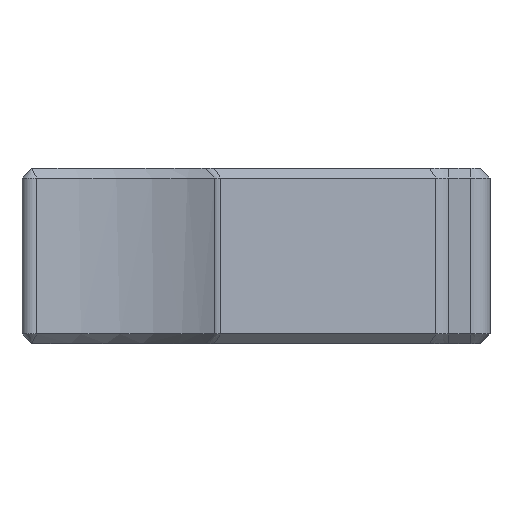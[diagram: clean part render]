
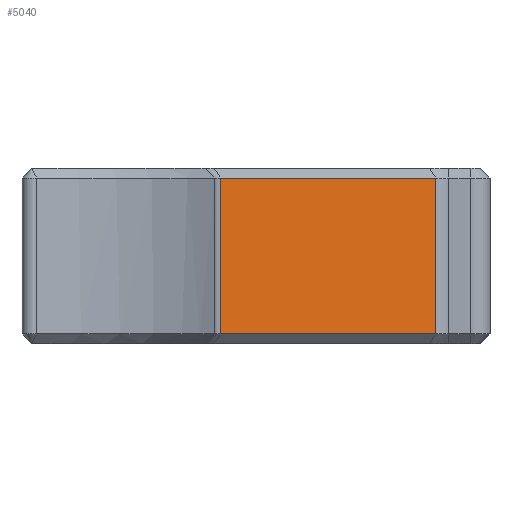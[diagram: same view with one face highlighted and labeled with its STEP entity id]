
A CAD part, front view. The second image highlights one B-rep face of the part: STEP entity #5040.
In plain terms, the highlighted planar face has unit normal (0.658, -0.753, 0).
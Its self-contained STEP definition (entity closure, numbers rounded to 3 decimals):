
#295 = VERTEX_POINT ( 'NONE', #6923 ) ;
#414 = EDGE_CURVE ( 'NONE', #295, #7731, #649, .T. ) ;
#551 = EDGE_LOOP ( 'NONE', ( #2454, #8305, #5130, #1067 ) ) ;
#649 = LINE ( 'NONE', #7793, #1592 ) ;
#946 = DIRECTION ( 'NONE',  ( -0.753, -0.658, 0. ) ) ;
#1033 = EDGE_CURVE ( 'NONE', #1755, #295, #6708, .T. ) ;
#1067 = ORIENTED_EDGE ( 'NONE', *, *, #8392, .T. ) ;
#1592 = VECTOR ( 'NONE', #3863, 1000. ) ;
#1755 = VERTEX_POINT ( 'NONE', #3009 ) ;
#1832 = CARTESIAN_POINT ( 'NONE',  ( 8.379, -9.581, -4. ) ) ;
#2094 = VECTOR ( 'NONE', #2822, 1000. ) ;
#2454 = ORIENTED_EDGE ( 'NONE', *, *, #7934, .T. ) ;
#2777 = DIRECTION ( 'NONE',  ( -0.658, 0.753, 0. ) ) ;
#2822 = DIRECTION ( 'NONE',  ( 0., 0., -1. ) ) ;
#3009 = CARTESIAN_POINT ( 'NONE',  ( 3.688, -13.683, -4. ) ) ;
#3605 = CARTESIAN_POINT ( 'NONE',  ( 3.688, -13.683, 4.5 ) ) ;
#3608 = CARTESIAN_POINT ( 'NONE',  ( 8.379, -9.581, 4.5 ) ) ;
#3863 = DIRECTION ( 'NONE',  ( 0., 0., 1. ) ) ;
#4887 = CARTESIAN_POINT ( 'NONE',  ( 3.688, -13.683, 4. ) ) ;
#5040 = ADVANCED_FACE ( 'NONE', ( #6718 ), #7538, .F. ) ;
#5047 = CARTESIAN_POINT ( 'NONE',  ( 14.717, -4.038, 4. ) ) ;
#5130 = ORIENTED_EDGE ( 'NONE', *, *, #414, .T. ) ;
#5161 = LINE ( 'NONE', #3605, #2094 ) ;
#5940 = CARTESIAN_POINT ( 'NONE',  ( 3.688, -13.683, 4. ) ) ;
#6605 = DIRECTION ( 'NONE',  ( 0.753, 0.658, 0. ) ) ;
#6708 = LINE ( 'NONE', #1832, #10175 ) ;
#6718 = FACE_OUTER_BOUND ( 'NONE', #551, .T. ) ;
#6923 = CARTESIAN_POINT ( 'NONE',  ( 14.717, -4.038, -4. ) ) ;
#7069 = LINE ( 'NONE', #4887, #8909 ) ;
#7391 = DIRECTION ( 'NONE',  ( -0.753, -0.658, 0. ) ) ;
#7538 = PLANE ( 'NONE',  #9439 ) ;
#7731 = VERTEX_POINT ( 'NONE', #5047 ) ;
#7793 = CARTESIAN_POINT ( 'NONE',  ( 14.717, -4.038, 4.5 ) ) ;
#7934 = EDGE_CURVE ( 'NONE', #7981, #1755, #5161, .T. ) ;
#7981 = VERTEX_POINT ( 'NONE', #5940 ) ;
#8305 = ORIENTED_EDGE ( 'NONE', *, *, #1033, .T. ) ;
#8392 = EDGE_CURVE ( 'NONE', #7731, #7981, #7069, .T. ) ;
#8909 = VECTOR ( 'NONE', #946, 1000. ) ;
#9439 = AXIS2_PLACEMENT_3D ( 'NONE', #3608, #2777, #7391 ) ;
#10175 = VECTOR ( 'NONE', #6605, 1000. ) ;
